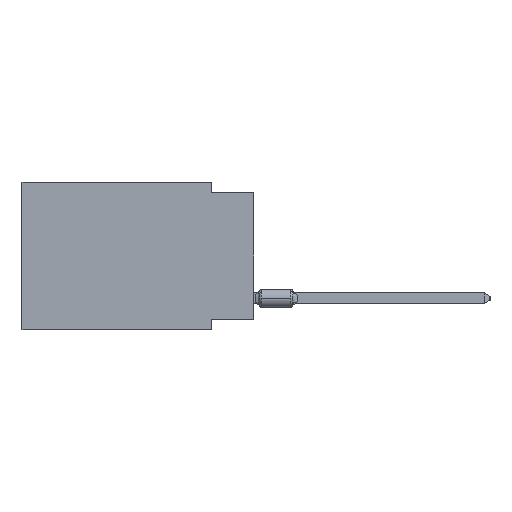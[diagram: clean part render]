
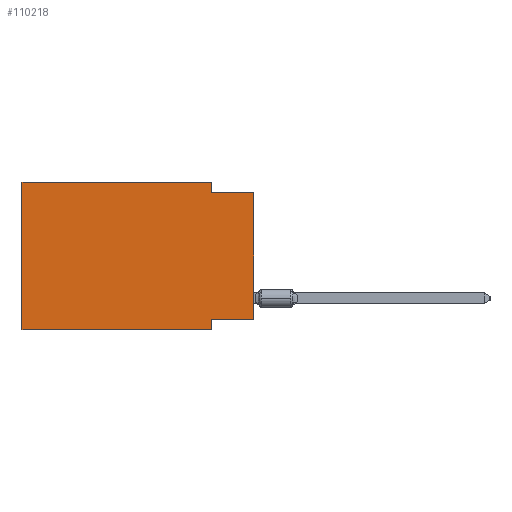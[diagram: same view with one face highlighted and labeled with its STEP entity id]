
A CAD part, left-side view. The second image highlights one B-rep face of the part: STEP entity #110218.
In plain terms, the highlighted planar face has unit normal (-1, 0, 0).
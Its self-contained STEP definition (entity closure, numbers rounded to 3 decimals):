
#222 = DIRECTION ( 'NONE',  ( 0., 0., 1. ) ) ;
#4138 = CARTESIAN_POINT ( 'NONE',  ( 0., 2.54, -8.255 ) ) ;
#4269 = EDGE_CURVE ( 'NONE', #76440, #9918, #109534, .T. ) ;
#4427 = LINE ( 'NONE', #30982, #7703 ) ;
#5726 = VERTEX_POINT ( 'NONE', #9593 ) ;
#7330 = LINE ( 'NONE', #53179, #53496 ) ;
#7703 = VECTOR ( 'NONE', #49670, 1000. ) ;
#7888 = VERTEX_POINT ( 'NONE', #106238 ) ;
#9593 = CARTESIAN_POINT ( 'NONE',  ( 0., 13.97, -8.89 ) ) ;
#9918 = VERTEX_POINT ( 'NONE', #19457 ) ;
#11728 = CARTESIAN_POINT ( 'NONE',  ( 0., 0., -0.635 ) ) ;
#15712 = VECTOR ( 'NONE', #112576, 1000. ) ;
#16008 = ORIENTED_EDGE ( 'NONE', *, *, #101940, .F. ) ;
#19457 = CARTESIAN_POINT ( 'NONE',  ( 0., 2.54, -0.635 ) ) ;
#19827 = EDGE_CURVE ( 'NONE', #5726, #36186, #4427, .T. ) ;
#20874 = FACE_OUTER_BOUND ( 'NONE', #118471, .T. ) ;
#21777 = VECTOR ( 'NONE', #222, 1000. ) ;
#23386 = EDGE_CURVE ( 'NONE', #7888, #24671, #95665, .T. ) ;
#24671 = VERTEX_POINT ( 'NONE', #4138 ) ;
#26155 = CARTESIAN_POINT ( 'NONE',  ( 0., 0., 0. ) ) ;
#30982 = CARTESIAN_POINT ( 'NONE',  ( 0., 13.97, -8.89 ) ) ;
#31848 = CARTESIAN_POINT ( 'NONE',  ( 0., 2.54, -8.89 ) ) ;
#34550 = DIRECTION ( 'NONE',  ( 0., -1., 0. ) ) ;
#36186 = VERTEX_POINT ( 'NONE', #31848 ) ;
#38438 = VECTOR ( 'NONE', #94223, 1000. ) ;
#42405 = CARTESIAN_POINT ( 'NONE',  ( 0., 0., -0.635 ) ) ;
#43505 = EDGE_CURVE ( 'NONE', #60645, #76440, #48141, .T. ) ;
#47548 = CARTESIAN_POINT ( 'NONE',  ( 0., 13.97, 0. ) ) ;
#47769 = LINE ( 'NONE', #84590, #38438 ) ;
#48141 = LINE ( 'NONE', #47548, #101133 ) ;
#49670 = DIRECTION ( 'NONE',  ( 0., -1., 0. ) ) ;
#53179 = CARTESIAN_POINT ( 'NONE',  ( 0., 2.54, -8.89 ) ) ;
#53496 = VECTOR ( 'NONE', #61654, 1000. ) ;
#54472 = CARTESIAN_POINT ( 'NONE',  ( 0., 13.97, 0. ) ) ;
#57663 = ORIENTED_EDGE ( 'NONE', *, *, #4269, .F. ) ;
#58283 = CARTESIAN_POINT ( 'NONE',  ( 0., 0., -8.255 ) ) ;
#58286 = PLANE ( 'NONE',  #68380 ) ;
#60645 = VERTEX_POINT ( 'NONE', #54472 ) ;
#61654 = DIRECTION ( 'NONE',  ( 0., 0., -1. ) ) ;
#64754 = LINE ( 'NONE', #26155, #21777 ) ;
#66118 = ORIENTED_EDGE ( 'NONE', *, *, #95376, .F. ) ;
#68380 = AXIS2_PLACEMENT_3D ( 'NONE', #96270, #76995, #103526 ) ;
#68427 = VECTOR ( 'NONE', #119164, 1000. ) ;
#76440 = VERTEX_POINT ( 'NONE', #100511 ) ;
#76824 = ORIENTED_EDGE ( 'NONE', *, *, #43505, .F. ) ;
#76995 = DIRECTION ( 'NONE',  ( 1., 0., 0. ) ) ;
#80971 = ORIENTED_EDGE ( 'NONE', *, *, #114588, .T. ) ;
#81953 = VECTOR ( 'NONE', #34550, 1000. ) ;
#84364 = DIRECTION ( 'NONE',  ( 0., -1., 0. ) ) ;
#84590 = CARTESIAN_POINT ( 'NONE',  ( 0., 13.97, 0. ) ) ;
#86319 = ORIENTED_EDGE ( 'NONE', *, *, #23386, .F. ) ;
#86412 = ORIENTED_EDGE ( 'NONE', *, *, #88830, .F. ) ;
#88830 = EDGE_CURVE ( 'NONE', #5726, #60645, #47769, .T. ) ;
#90046 = LINE ( 'NONE', #42405, #81953 ) ;
#94223 = DIRECTION ( 'NONE',  ( 0., 0., 1. ) ) ;
#95376 = EDGE_CURVE ( 'NONE', #9918, #96391, #90046, .T. ) ;
#95665 = LINE ( 'NONE', #58283, #15712 ) ;
#96270 = CARTESIAN_POINT ( 'NONE',  ( 0., 13.97, 0. ) ) ;
#96391 = VERTEX_POINT ( 'NONE', #11728 ) ;
#100511 = CARTESIAN_POINT ( 'NONE',  ( 0., 2.54, 0. ) ) ;
#101071 = CARTESIAN_POINT ( 'NONE',  ( 0., 2.54, 0. ) ) ;
#101133 = VECTOR ( 'NONE', #84364, 1000. ) ;
#101940 = EDGE_CURVE ( 'NONE', #24671, #36186, #7330, .T. ) ;
#103526 = DIRECTION ( 'NONE',  ( 0., 0., -1. ) ) ;
#106238 = CARTESIAN_POINT ( 'NONE',  ( 0., 0., -8.255 ) ) ;
#109534 = LINE ( 'NONE', #101071, #68427 ) ;
#110218 = ADVANCED_FACE ( 'NONE', ( #20874 ), #58286, .F. ) ;
#112576 = DIRECTION ( 'NONE',  ( 0., 1., 0. ) ) ;
#114588 = EDGE_CURVE ( 'NONE', #7888, #96391, #64754, .T. ) ;
#118471 = EDGE_LOOP ( 'NONE', ( #80971, #66118, #57663, #76824, #86412, #118914, #16008, #86319 ) ) ;
#118914 = ORIENTED_EDGE ( 'NONE', *, *, #19827, .T. ) ;
#119164 = DIRECTION ( 'NONE',  ( 0., 0., -1. ) ) ;
